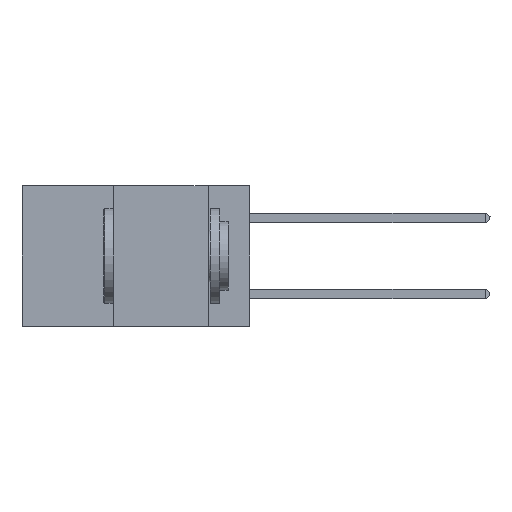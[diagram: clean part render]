
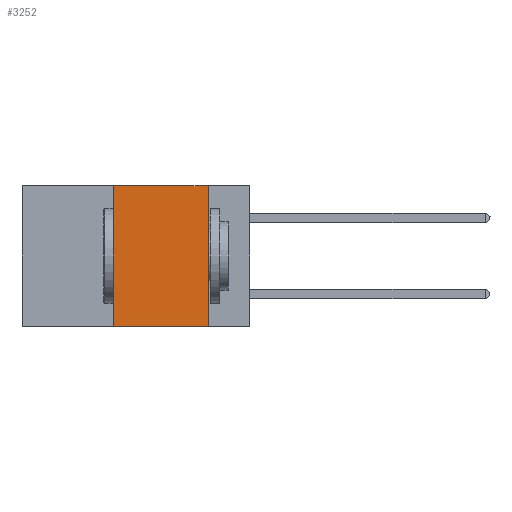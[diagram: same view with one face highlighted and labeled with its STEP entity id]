
A CAD part, left-side view. The second image highlights one B-rep face of the part: STEP entity #3252.
In plain terms, the highlighted planar face has unit normal (-1, 0, 0).
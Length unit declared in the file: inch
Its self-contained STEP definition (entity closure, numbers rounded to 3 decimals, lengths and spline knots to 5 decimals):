
#13 = VECTOR ( 'NONE', #1750, 39.37008 ) ;
#22 = VECTOR ( 'NONE', #2186, 39.37008 ) ;
#877 = EDGE_CURVE ( 'NONE', #2440, #9085, #9294, .T. ) ;
#1412 = CARTESIAN_POINT ( 'NONE',  ( 0., 0.11, -0.37 ) ) ;
#1750 = DIRECTION ( 'NONE',  ( 0., 0., -1. ) ) ;
#1890 = LINE ( 'NONE', #8917, #13 ) ;
#1970 = CARTESIAN_POINT ( 'NONE',  ( 0., 0.6, 0. ) ) ;
#2073 = EDGE_CURVE ( 'NONE', #2440, #8131, #5027, .T. ) ;
#2186 = DIRECTION ( 'NONE',  ( 0., -1., 0. ) ) ;
#2255 = CARTESIAN_POINT ( 'NONE',  ( 0., 0.36, 0. ) ) ;
#2440 = VERTEX_POINT ( 'NONE', #3227 ) ;
#2893 = VECTOR ( 'NONE', #9514, 39.37008 ) ;
#3227 = CARTESIAN_POINT ( 'NONE',  ( 0., 0.36, -0.37 ) ) ;
#3252 = ADVANCED_FACE ( 'NONE', ( #7661 ), #9181, .F. ) ;
#3609 = ORIENTED_EDGE ( 'NONE', *, *, #2073, .F. ) ;
#3683 = VERTEX_POINT ( 'NONE', #5508 ) ;
#5027 = LINE ( 'NONE', #10340, #2893 ) ;
#5049 = ORIENTED_EDGE ( 'NONE', *, *, #877, .T. ) ;
#5136 = DIRECTION ( 'NONE',  ( 1., 0., 0. ) ) ;
#5427 = CARTESIAN_POINT ( 'NONE',  ( 0., 0.6, 0. ) ) ;
#5432 = LINE ( 'NONE', #5427, #22 ) ;
#5508 = CARTESIAN_POINT ( 'NONE',  ( 0., 0.11, 0. ) ) ;
#5780 = ORIENTED_EDGE ( 'NONE', *, *, #9872, .F. ) ;
#5859 = ORIENTED_EDGE ( 'NONE', *, *, #9622, .F. ) ;
#6717 = DIRECTION ( 'NONE',  ( 0., 0., -1. ) ) ;
#6792 = CARTESIAN_POINT ( 'NONE',  ( 0., 0.6, -0.37 ) ) ;
#7608 = DIRECTION ( 'NONE',  ( 0., -1., 0. ) ) ;
#7639 = AXIS2_PLACEMENT_3D ( 'NONE', #1970, #5136, #6717 ) ;
#7661 = FACE_OUTER_BOUND ( 'NONE', #7996, .T. ) ;
#7996 = EDGE_LOOP ( 'NONE', ( #5780, #5859, #3609, #5049 ) ) ;
#8131 = VERTEX_POINT ( 'NONE', #2255 ) ;
#8917 = CARTESIAN_POINT ( 'NONE',  ( 0., 0.11, 0. ) ) ;
#9085 = VERTEX_POINT ( 'NONE', #1412 ) ;
#9181 = PLANE ( 'NONE',  #7639 ) ;
#9294 = LINE ( 'NONE', #6792, #10173 ) ;
#9514 = DIRECTION ( 'NONE',  ( 0., 0., 1. ) ) ;
#9622 = EDGE_CURVE ( 'NONE', #8131, #3683, #5432, .T. ) ;
#9872 = EDGE_CURVE ( 'NONE', #3683, #9085, #1890, .T. ) ;
#10173 = VECTOR ( 'NONE', #7608, 39.37008 ) ;
#10340 = CARTESIAN_POINT ( 'NONE',  ( 0., 0.36, 0. ) ) ;
